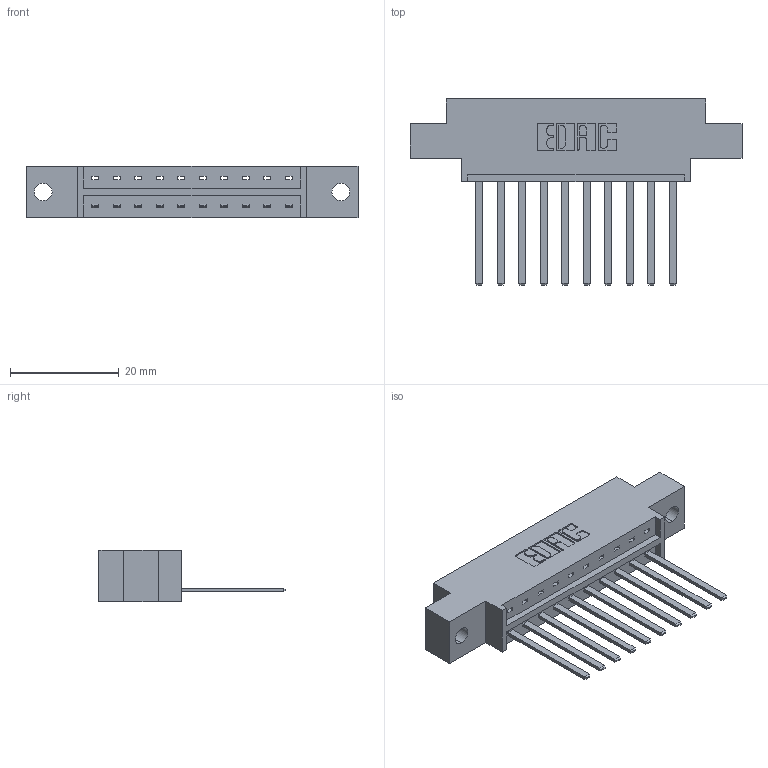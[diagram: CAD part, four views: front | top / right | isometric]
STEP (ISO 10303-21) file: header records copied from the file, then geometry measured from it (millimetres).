
FILE_DESCRIPTION (( 'STEP AP203' ), '1' );
FILE_NAME ('333-010-544-602.STEP', '2018-07-31T23:06:41', ( '' ), ( '' ), 'SwSTEP 2.0', 'SolidWorks 2016', '' );
FILE_SCHEMA (( 'CONFIG_CONTROL_DESIGN' ));
Length unit declared in the file: inch
Products named in the file (3): 333 Part_Offset - .128 Dia; 345-292-001_345-293-144; 333-010-544-602
Assembly tree (11 placements, depth 2):
  333-010-544-602
    333 Part_Offset - .128 Dia
    345-292-001_345-293-144  x10
Bounding box: 61.16 x 34.3 x 9.4 mm (x, y, z)
Volume: 5730.9 mm3; surface area: 6293.6 mm2
Topology: 11 solids, 11 shells, 638 faces, 1903 edges, 1254 vertices
Faces by surface type: plane 454, cylinder 184
Entity records: 10203 total; most frequent: CARTESIAN_POINT 1772, ORIENTED_EDGE 1718, DIRECTION 1555, EDGE_CURVE 859, VECTOR 735, LINE 735, VERTEX_POINT 570, AXIS2_PLACEMENT_3D 410
